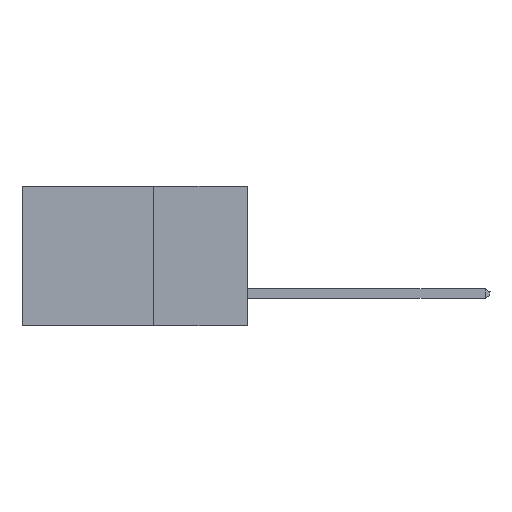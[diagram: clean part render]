
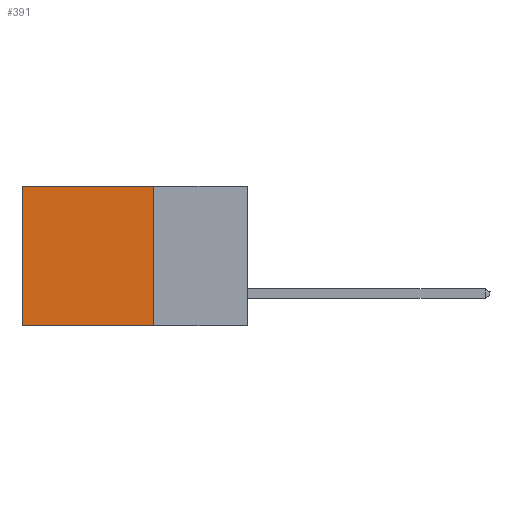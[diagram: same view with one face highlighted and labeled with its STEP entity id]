
A CAD part, left-side view. The second image highlights one B-rep face of the part: STEP entity #391.
In plain terms, the highlighted planar face has unit normal (-1, 0, 0).
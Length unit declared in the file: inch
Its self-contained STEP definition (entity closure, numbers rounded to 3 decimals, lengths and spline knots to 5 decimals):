
#327 = VERTEX_POINT ( 'NONE', #10502 ) ;
#391 = ADVANCED_FACE ( 'NONE', ( #11542 ), #1214, .F. ) ;
#457 = CARTESIAN_POINT ( 'NONE',  ( 0.2615, 0.6, 0. ) ) ;
#852 = VERTEX_POINT ( 'NONE', #457 ) ;
#1179 = VECTOR ( 'NONE', #12031, 39.37008 ) ;
#1214 = PLANE ( 'NONE',  #2442 ) ;
#1788 = DIRECTION ( 'NONE',  ( 0., 0., -1. ) ) ;
#2229 = LINE ( 'NONE', #16521, #15597 ) ;
#2442 = AXIS2_PLACEMENT_3D ( 'NONE', #6313, #10346, #3802 ) ;
#2445 = ORIENTED_EDGE ( 'NONE', *, *, #4218, .T. ) ;
#3802 = DIRECTION ( 'NONE',  ( 0., 0., -1. ) ) ;
#4218 = EDGE_CURVE ( 'NONE', #852, #15655, #11330, .T. ) ;
#4760 = ORIENTED_EDGE ( 'NONE', *, *, #6934, .F. ) ;
#4891 = DIRECTION ( 'NONE',  ( 0., 1., 0. ) ) ;
#5654 = CARTESIAN_POINT ( 'NONE',  ( 0.2615, 0.6, -0.37 ) ) ;
#6313 = CARTESIAN_POINT ( 'NONE',  ( 0.2615, 0.25, -0.37 ) ) ;
#6934 = EDGE_CURVE ( 'NONE', #327, #12223, #7764, .T. ) ;
#7007 = VECTOR ( 'NONE', #4891, 39.37008 ) ;
#7764 = LINE ( 'NONE', #10576, #1179 ) ;
#9968 = DIRECTION ( 'NONE',  ( 0., 1., 0. ) ) ;
#10346 = DIRECTION ( 'NONE',  ( 1., 0., 0. ) ) ;
#10502 = CARTESIAN_POINT ( 'NONE',  ( 0.2615, 0.25, 0. ) ) ;
#10576 = CARTESIAN_POINT ( 'NONE',  ( 0.2615, 0.25, -0.37 ) ) ;
#11065 = CARTESIAN_POINT ( 'NONE',  ( 0.2615, 0.6, -0.37 ) ) ;
#11330 = LINE ( 'NONE', #11065, #16018 ) ;
#11542 = FACE_OUTER_BOUND ( 'NONE', #16913, .T. ) ;
#12031 = DIRECTION ( 'NONE',  ( 0., 0., -1. ) ) ;
#12223 = VERTEX_POINT ( 'NONE', #13781 ) ;
#12735 = LINE ( 'NONE', #16698, #7007 ) ;
#12942 = EDGE_CURVE ( 'NONE', #327, #852, #2229, .T. ) ;
#13167 = ORIENTED_EDGE ( 'NONE', *, *, #12942, .T. ) ;
#13509 = ORIENTED_EDGE ( 'NONE', *, *, #14218, .F. ) ;
#13781 = CARTESIAN_POINT ( 'NONE',  ( 0.2615, 0.25, -0.37 ) ) ;
#14218 = EDGE_CURVE ( 'NONE', #12223, #15655, #12735, .T. ) ;
#15597 = VECTOR ( 'NONE', #9968, 39.37008 ) ;
#15655 = VERTEX_POINT ( 'NONE', #5654 ) ;
#16018 = VECTOR ( 'NONE', #1788, 39.37008 ) ;
#16521 = CARTESIAN_POINT ( 'NONE',  ( 0.2615, 0.25, 0. ) ) ;
#16698 = CARTESIAN_POINT ( 'NONE',  ( 0.2615, 0.25, -0.37 ) ) ;
#16913 = EDGE_LOOP ( 'NONE', ( #2445, #13509, #4760, #13167 ) ) ;
